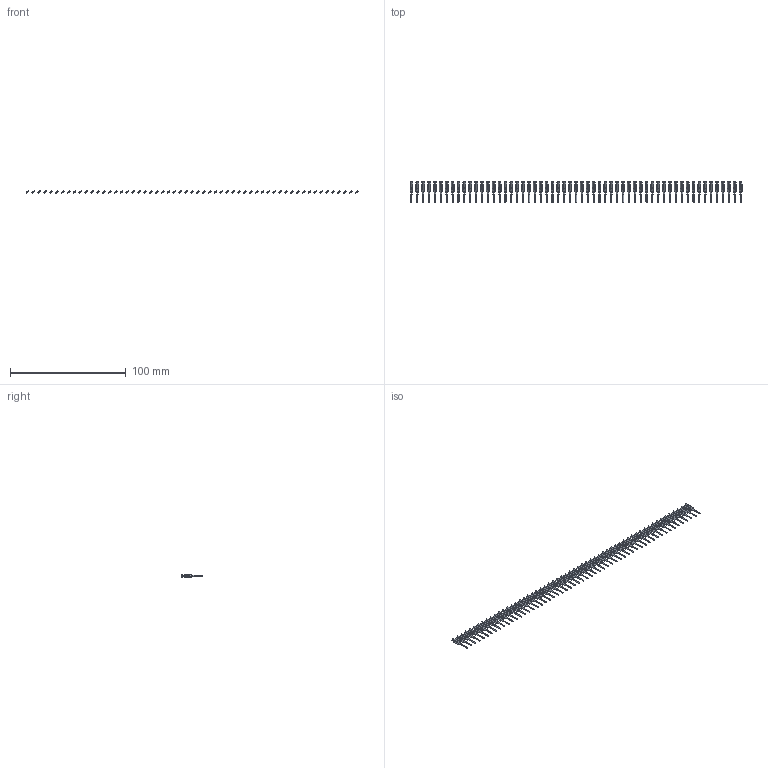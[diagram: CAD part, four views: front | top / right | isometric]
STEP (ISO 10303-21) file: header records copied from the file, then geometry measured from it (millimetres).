
FILE_DESCRIPTION (( 'STEP AP203' ), '1' );
FILE_NAME ('106-057-251-200.STEP', '2020-04-16T20:43:54', ( '' ), ( '' ), 'SwSTEP 2.0', 'SolidWorks 2016', '' );
FILE_SCHEMA (( 'CONFIG_CONTROL_DESIGN' ));
Length unit declared in the file: inch
Products named in the file (2): 106-057-251-200; 100-290-001_100-290-251
Assembly tree (57 placements, depth 2):
  106-057-251-200
    100-290-001_100-290-251  x57
Bounding box: 287.01 x 17.9 x 2.53 mm (x, y, z)
Volume: 1042.2 mm3; surface area: 5122.5 mm2
Topology: 57 solids, 57 shells, 1596 faces, 4446 edges, 2964 vertices
Faces by surface type: plane 1254, cylinder 342
Entity records: 2886 total; most frequent: DIRECTION 262, CARTESIAN_POINT 230, ORIENTED_EDGE 156, COORDINATED_UNIVERSAL_TIME_OFFSET 124, LOCAL_TIME 124, CALENDAR_DATE 124, DATE_AND_TIME 124, AXIS2_PLACEMENT_3D 100
